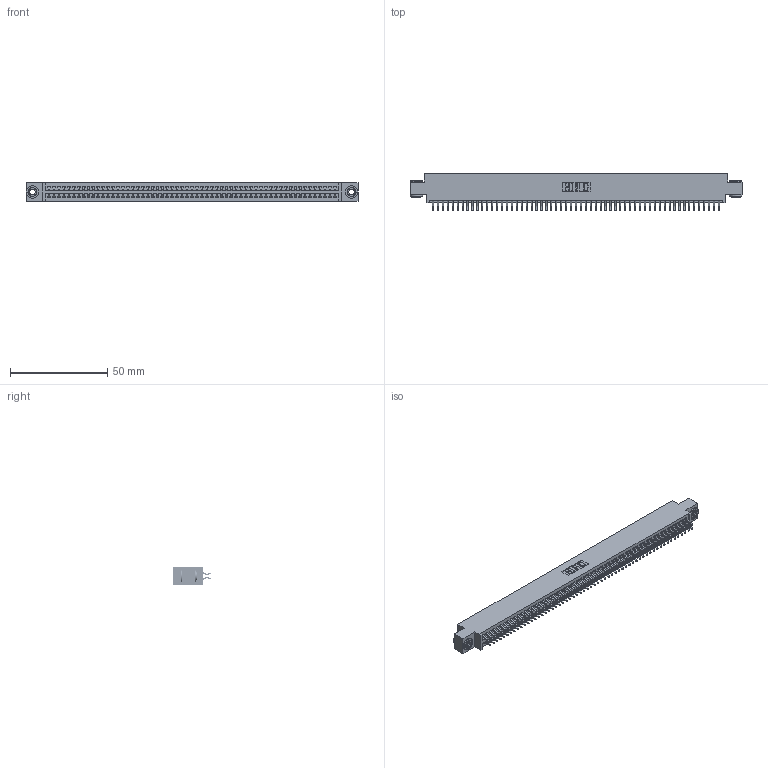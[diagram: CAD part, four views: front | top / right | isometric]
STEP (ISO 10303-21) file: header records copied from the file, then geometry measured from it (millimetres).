
FILE_DESCRIPTION (( 'STEP AP203' ), '1' );
FILE_NAME ('395-118-556-803.STEP', '2019-10-28T02:45:16', ( '' ), ( '' ), 'SwSTEP 2.0', 'SolidWorks 2016', '' );
FILE_SCHEMA (( 'CONFIG_CONTROL_DESIGN' ));
Length unit declared in the file: inch
Products named in the file (4): 345-250-002_345-250-002-102; 395-118-556-803; 345 Part_0.170 Offset - 0.156 Dia-TH; 345-292-001_556 Tail
Assembly tree (121 placements, depth 2):
  395-118-556-803
    345 Part_0.170 Offset - 0.156 Dia-TH
    345-292-001_556 Tail  x118
    345-250-002_345-250-002-102  x2
Bounding box: 171.07 x 19.24 x 9.4 mm (x, y, z)
Volume: 16677 mm3; surface area: 25225.7 mm2
Topology: 121 solids, 121 shells, 6776 faces, 20135 edges, 13262 vertices
Faces by surface type: plane 4460, cylinder 2308, cone 8
Entity records: 45006 total; most frequent: CARTESIAN_POINT 7519, ORIENTED_EDGE 7434, DIRECTION 6627, EDGE_CURVE 3717, VECTOR 3317, LINE 3317, VERTEX_POINT 2474, AXIS2_PLACEMENT_3D 1655
